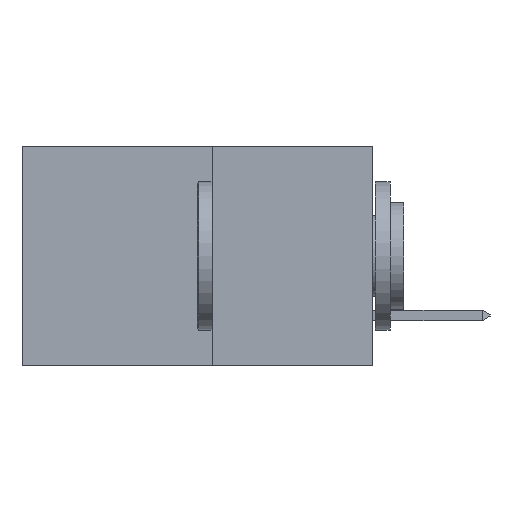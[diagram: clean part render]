
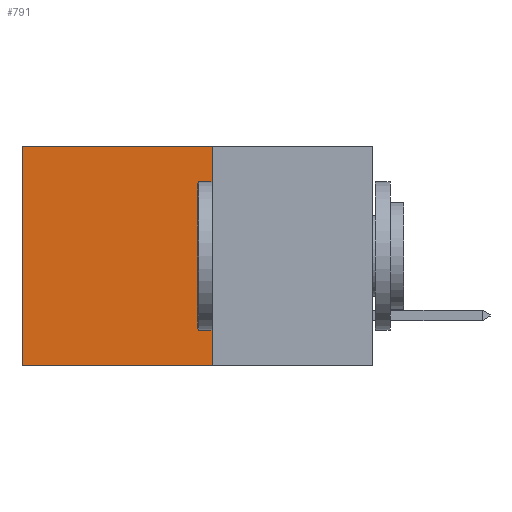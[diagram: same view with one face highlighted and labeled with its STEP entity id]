
A CAD part, left-side view. The second image highlights one B-rep face of the part: STEP entity #791.
In plain terms, the highlighted planar face has unit normal (-1, 0, 0).
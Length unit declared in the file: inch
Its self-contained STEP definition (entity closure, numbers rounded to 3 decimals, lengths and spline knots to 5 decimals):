
#595 = CARTESIAN_POINT ( 'NONE',  ( 0.277, 0.59, -0.37 ) ) ;
#791 = ADVANCED_FACE ( 'NONE', ( #19670 ), #20164, .F. ) ;
#2347 = LINE ( 'NONE', #26574, #13434 ) ;
#3402 = DIRECTION ( 'NONE',  ( 1., 0., 0. ) ) ;
#3425 = CARTESIAN_POINT ( 'NONE',  ( 0.277, 0.27, -0.37 ) ) ;
#3732 = DIRECTION ( 'NONE',  ( 0., 1., 0. ) ) ;
#5587 = VERTEX_POINT ( 'NONE', #6111 ) ;
#5835 = CARTESIAN_POINT ( 'NONE',  ( 0.277, 0.27, -0.37 ) ) ;
#6111 = CARTESIAN_POINT ( 'NONE',  ( 0.277, 0.59, 0. ) ) ;
#6397 = EDGE_CURVE ( 'NONE', #17869, #24861, #2347, .T. ) ;
#10095 = DIRECTION ( 'NONE',  ( 0., 0., -1. ) ) ;
#12580 = CARTESIAN_POINT ( 'NONE',  ( 0.277, 0.27, -0.37 ) ) ;
#12791 = VERTEX_POINT ( 'NONE', #17969 ) ;
#12875 = CARTESIAN_POINT ( 'NONE',  ( 0.277, 0.59, -0.37 ) ) ;
#13434 = VECTOR ( 'NONE', #15485, 39.37008 ) ;
#13991 = VECTOR ( 'NONE', #25860, 39.37008 ) ;
#15485 = DIRECTION ( 'NONE',  ( 0., 1., 0. ) ) ;
#15680 = ORIENTED_EDGE ( 'NONE', *, *, #19966, .F. ) ;
#15848 = VECTOR ( 'NONE', #21859, 39.37008 ) ;
#17865 = VECTOR ( 'NONE', #3732, 39.37008 ) ;
#17869 = VERTEX_POINT ( 'NONE', #12580 ) ;
#17969 = CARTESIAN_POINT ( 'NONE',  ( 0.277, 0.27, 0. ) ) ;
#19281 = CARTESIAN_POINT ( 'NONE',  ( 0.277, 0.27, 0. ) ) ;
#19670 = FACE_OUTER_BOUND ( 'NONE', #25087, .T. ) ;
#19966 = EDGE_CURVE ( 'NONE', #12791, #17869, #25851, .T. ) ;
#20164 = PLANE ( 'NONE',  #21452 ) ;
#21452 = AXIS2_PLACEMENT_3D ( 'NONE', #3425, #3402, #10095 ) ;
#21780 = LINE ( 'NONE', #12875, #15848 ) ;
#21859 = DIRECTION ( 'NONE',  ( 0., 0., -1. ) ) ;
#23072 = LINE ( 'NONE', #19281, #17865 ) ;
#23880 = ORIENTED_EDGE ( 'NONE', *, *, #28176, .T. ) ;
#24597 = EDGE_CURVE ( 'NONE', #12791, #5587, #23072, .T. ) ;
#24861 = VERTEX_POINT ( 'NONE', #595 ) ;
#25087 = EDGE_LOOP ( 'NONE', ( #23880, #26136, #15680, #26496 ) ) ;
#25851 = LINE ( 'NONE', #5835, #13991 ) ;
#25860 = DIRECTION ( 'NONE',  ( 0., 0., -1. ) ) ;
#26136 = ORIENTED_EDGE ( 'NONE', *, *, #6397, .F. ) ;
#26496 = ORIENTED_EDGE ( 'NONE', *, *, #24597, .T. ) ;
#26574 = CARTESIAN_POINT ( 'NONE',  ( 0.277, 0.27, -0.37 ) ) ;
#28176 = EDGE_CURVE ( 'NONE', #5587, #24861, #21780, .T. ) ;
